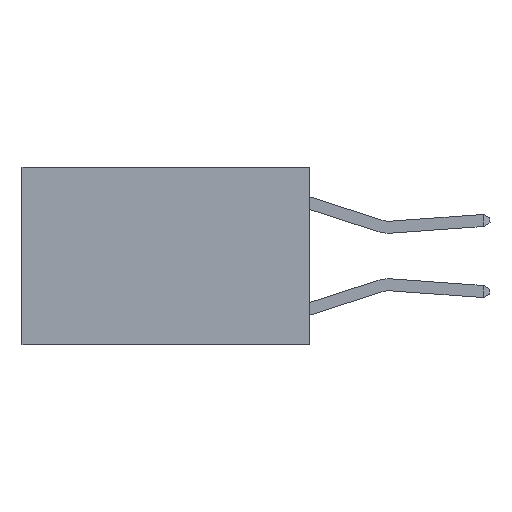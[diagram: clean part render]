
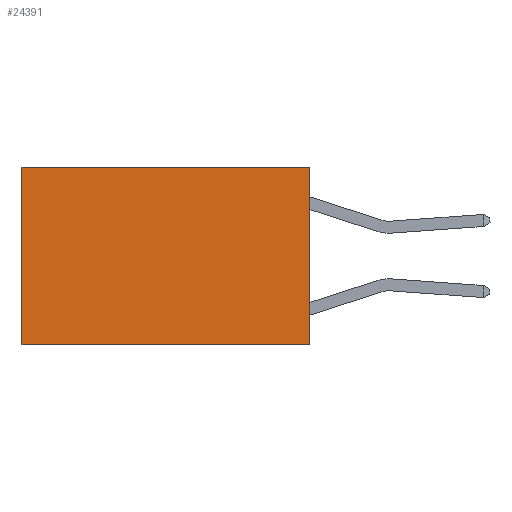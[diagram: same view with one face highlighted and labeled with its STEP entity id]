
A CAD part, left-side view. The second image highlights one B-rep face of the part: STEP entity #24391.
In plain terms, the highlighted planar face has unit normal (-1, 0, 0).
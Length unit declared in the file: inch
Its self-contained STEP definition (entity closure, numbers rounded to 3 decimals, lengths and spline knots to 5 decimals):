
#496 = LINE ( 'NONE', #9846, #5357 ) ;
#1910 = CARTESIAN_POINT ( 'NONE',  ( 0.2625, 0., -0.37 ) ) ;
#4246 = VECTOR ( 'NONE', #26440, 39.37008 ) ;
#4524 = AXIS2_PLACEMENT_3D ( 'NONE', #14200, #9571, #7479 ) ;
#5241 = ORIENTED_EDGE ( 'NONE', *, *, #12858, .F. ) ;
#5357 = VECTOR ( 'NONE', #25482, 39.37008 ) ;
#5729 = CARTESIAN_POINT ( 'NONE',  ( 0.2625, 0., 0. ) ) ;
#6141 = ORIENTED_EDGE ( 'NONE', *, *, #19571, .F. ) ;
#6188 = EDGE_LOOP ( 'NONE', ( #11254, #5241, #6141, #9558 ) ) ;
#7479 = DIRECTION ( 'NONE',  ( 0., 0., -1. ) ) ;
#8327 = VERTEX_POINT ( 'NONE', #24280 ) ;
#8502 = EDGE_CURVE ( 'NONE', #28702, #10461, #20205, .T. ) ;
#8828 = DIRECTION ( 'NONE',  ( 0., 1., 0. ) ) ;
#9279 = FACE_OUTER_BOUND ( 'NONE', #6188, .T. ) ;
#9375 = CARTESIAN_POINT ( 'NONE',  ( 0.2625, 0., 0. ) ) ;
#9558 = ORIENTED_EDGE ( 'NONE', *, *, #18233, .T. ) ;
#9571 = DIRECTION ( 'NONE',  ( 1., 0., 0. ) ) ;
#9846 = CARTESIAN_POINT ( 'NONE',  ( 0.2625, 0., 0. ) ) ;
#10215 = LINE ( 'NONE', #5729, #4246 ) ;
#10461 = VERTEX_POINT ( 'NONE', #14082 ) ;
#11254 = ORIENTED_EDGE ( 'NONE', *, *, #8502, .T. ) ;
#12858 = EDGE_CURVE ( 'NONE', #8327, #10461, #25795, .T. ) ;
#14004 = DIRECTION ( 'NONE',  ( 0., 0., -1. ) ) ;
#14072 = VERTEX_POINT ( 'NONE', #9375 ) ;
#14082 = CARTESIAN_POINT ( 'NONE',  ( 0.2625, 0.6, -0.37 ) ) ;
#14200 = CARTESIAN_POINT ( 'NONE',  ( 0.2625, 0., 0. ) ) ;
#18233 = EDGE_CURVE ( 'NONE', #14072, #28702, #496, .T. ) ;
#18583 = VECTOR ( 'NONE', #8828, 39.37008 ) ;
#18635 = CARTESIAN_POINT ( 'NONE',  ( 0.2625, 0.6, 0. ) ) ;
#19571 = EDGE_CURVE ( 'NONE', #14072, #8327, #10215, .T. ) ;
#20205 = LINE ( 'NONE', #24665, #25365 ) ;
#24280 = CARTESIAN_POINT ( 'NONE',  ( 0.2625, 0., -0.37 ) ) ;
#24391 = ADVANCED_FACE ( 'NONE', ( #9279 ), #27040, .F. ) ;
#24665 = CARTESIAN_POINT ( 'NONE',  ( 0.2625, 0.6, 0. ) ) ;
#25365 = VECTOR ( 'NONE', #14004, 39.37008 ) ;
#25482 = DIRECTION ( 'NONE',  ( 0., 1., 0. ) ) ;
#25795 = LINE ( 'NONE', #1910, #18583 ) ;
#26440 = DIRECTION ( 'NONE',  ( 0., 0., -1. ) ) ;
#27040 = PLANE ( 'NONE',  #4524 ) ;
#28702 = VERTEX_POINT ( 'NONE', #18635 ) ;
